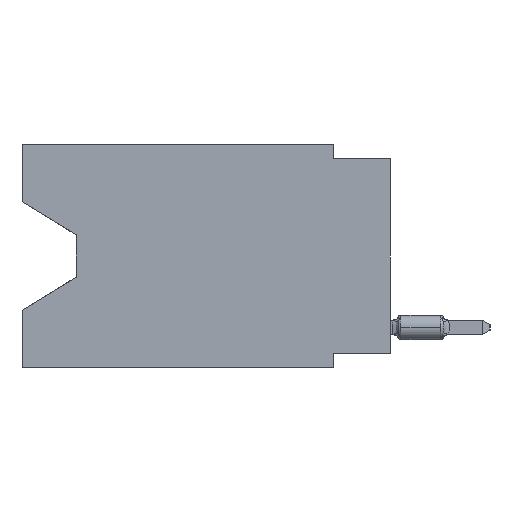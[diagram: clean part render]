
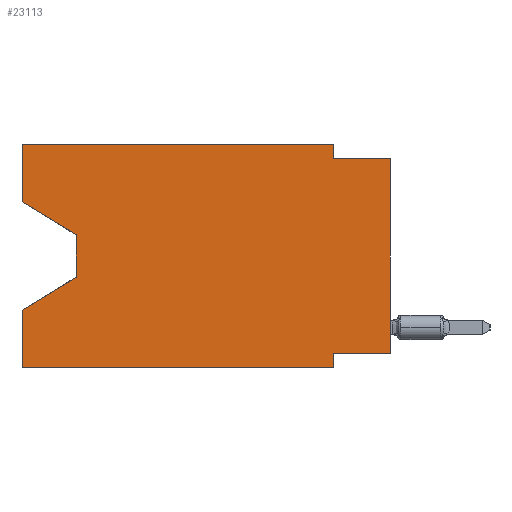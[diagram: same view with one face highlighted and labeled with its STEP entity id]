
A CAD part, left-side view. The second image highlights one B-rep face of the part: STEP entity #23113.
In plain terms, the highlighted planar face has unit normal (-1, 0, 0).
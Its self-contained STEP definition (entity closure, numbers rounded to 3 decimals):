
#590 = VECTOR ( 'NONE', #9091, 1000. ) ;
#1572 = VERTEX_POINT ( 'NONE', #11449 ) ;
#1670 = LINE ( 'NONE', #17598, #19760 ) ;
#2227 = CARTESIAN_POINT ( 'NONE',  ( 0., 0., 0. ) ) ;
#2711 = VECTOR ( 'NONE', #23779, 1000. ) ;
#2842 = DIRECTION ( 'NONE',  ( 0., -1., 0. ) ) ;
#3525 = LINE ( 'NONE', #7686, #2711 ) ;
#3571 = DIRECTION ( 'NONE',  ( 0., 0., -1. ) ) ;
#3828 = ORIENTED_EDGE ( 'NONE', *, *, #14545, .F. ) ;
#3966 = DIRECTION ( 'NONE',  ( 0., 0., 1. ) ) ;
#4262 = EDGE_CURVE ( 'NONE', #13019, #16238, #15889, .T. ) ;
#4271 = CARTESIAN_POINT ( 'NONE',  ( 0., 16.383, -2.546 ) ) ;
#4571 = CARTESIAN_POINT ( 'NONE',  ( 0., 2.54, 0. ) ) ;
#4600 = EDGE_CURVE ( 'NONE', #20387, #22314, #3525, .T. ) ;
#4717 = CARTESIAN_POINT ( 'NONE',  ( 0., 0., -9.271 ) ) ;
#4892 = EDGE_LOOP ( 'NONE', ( #18531, #23934, #24945, #11425, #24817, #5086, #17819, #14226, #20043, #3828, #9235, #13621 ) ) ;
#5086 = ORIENTED_EDGE ( 'NONE', *, *, #4600, .F. ) ;
#5108 = DIRECTION ( 'NONE',  ( 0., 0., -1. ) ) ;
#5160 = CARTESIAN_POINT ( 'NONE',  ( 0., 2.54, -0.635 ) ) ;
#5373 = EDGE_CURVE ( 'NONE', #19283, #24603, #5994, .T. ) ;
#5994 = LINE ( 'NONE', #12174, #19385 ) ;
#5995 = CARTESIAN_POINT ( 'NONE',  ( 0., 16.383, -9.906 ) ) ;
#6090 = LINE ( 'NONE', #13865, #24617 ) ;
#6990 = PLANE ( 'NONE',  #14774 ) ;
#7365 = CARTESIAN_POINT ( 'NONE',  ( 0., 0., -0.635 ) ) ;
#7686 = CARTESIAN_POINT ( 'NONE',  ( 0., 2.54, -9.906 ) ) ;
#8246 = LINE ( 'NONE', #12695, #17704 ) ;
#8514 = VERTEX_POINT ( 'NONE', #7365 ) ;
#8812 = VECTOR ( 'NONE', #2842, 1000. ) ;
#9091 = DIRECTION ( 'NONE',  ( 0., 0., -1. ) ) ;
#9235 = ORIENTED_EDGE ( 'NONE', *, *, #19040, .F. ) ;
#9449 = CARTESIAN_POINT ( 'NONE',  ( 0., 16.383, 0. ) ) ;
#9459 = CARTESIAN_POINT ( 'NONE',  ( 0., 16.383, -9.906 ) ) ;
#9514 = VERTEX_POINT ( 'NONE', #24163 ) ;
#9775 = CARTESIAN_POINT ( 'NONE',  ( 0., 16.383, 0. ) ) ;
#9853 = EDGE_CURVE ( 'NONE', #26405, #9514, #11946, .T. ) ;
#9972 = CARTESIAN_POINT ( 'NONE',  ( 0., 2.54, -9.271 ) ) ;
#10276 = EDGE_CURVE ( 'NONE', #10586, #8514, #21690, .T. ) ;
#10586 = VERTEX_POINT ( 'NONE', #5160 ) ;
#11425 = ORIENTED_EDGE ( 'NONE', *, *, #9853, .F. ) ;
#11449 = CARTESIAN_POINT ( 'NONE',  ( 0., 2.54, 0. ) ) ;
#11501 = LINE ( 'NONE', #9459, #8812 ) ;
#11634 = VECTOR ( 'NONE', #23858, 1000. ) ;
#11694 = CARTESIAN_POINT ( 'NONE',  ( 0., 0., -9.271 ) ) ;
#11946 = LINE ( 'NONE', #9775, #11634 ) ;
#12174 = CARTESIAN_POINT ( 'NONE',  ( 0., 13.97, -4.013 ) ) ;
#12695 = CARTESIAN_POINT ( 'NONE',  ( 0., 16.383, -2.546 ) ) ;
#12700 = VECTOR ( 'NONE', #3966, 1000. ) ;
#13019 = VERTEX_POINT ( 'NONE', #4271 ) ;
#13621 = ORIENTED_EDGE ( 'NONE', *, *, #4262, .F. ) ;
#13865 = CARTESIAN_POINT ( 'NONE',  ( 0., 16.383, 0. ) ) ;
#14111 = EDGE_CURVE ( 'NONE', #13019, #19283, #8246, .T. ) ;
#14156 = LINE ( 'NONE', #2227, #12700 ) ;
#14226 = ORIENTED_EDGE ( 'NONE', *, *, #24074, .T. ) ;
#14545 = EDGE_CURVE ( 'NONE', #1572, #10586, #23308, .T. ) ;
#14774 = AXIS2_PLACEMENT_3D ( 'NONE', #25496, #23464, #5108 ) ;
#15572 = LINE ( 'NONE', #11694, #23337 ) ;
#15725 = VERTEX_POINT ( 'NONE', #4717 ) ;
#15889 = LINE ( 'NONE', #9449, #21069 ) ;
#15907 = DIRECTION ( 'NONE',  ( 0., -1., 0. ) ) ;
#16046 = DIRECTION ( 'NONE',  ( 0., 0., 1. ) ) ;
#16238 = VERTEX_POINT ( 'NONE', #25583 ) ;
#16348 = VECTOR ( 'NONE', #15907, 1000. ) ;
#17598 = CARTESIAN_POINT ( 'NONE',  ( 0., 13.97, -5.893 ) ) ;
#17704 = VECTOR ( 'NONE', #22990, 1000. ) ;
#17819 = ORIENTED_EDGE ( 'NONE', *, *, #19540, .F. ) ;
#17880 = DIRECTION ( 'NONE',  ( 0., -1., 0. ) ) ;
#18502 = CARTESIAN_POINT ( 'NONE',  ( 0., 13.97, -5.893 ) ) ;
#18531 = ORIENTED_EDGE ( 'NONE', *, *, #14111, .T. ) ;
#19040 = EDGE_CURVE ( 'NONE', #16238, #1572, #6090, .T. ) ;
#19080 = CARTESIAN_POINT ( 'NONE',  ( 0., 13.97, -4.013 ) ) ;
#19283 = VERTEX_POINT ( 'NONE', #19080 ) ;
#19385 = VECTOR ( 'NONE', #3571, 1000. ) ;
#19540 = EDGE_CURVE ( 'NONE', #15725, #20387, #15572, .T. ) ;
#19611 = DIRECTION ( 'NONE',  ( 0., 0.855, -0.519 ) ) ;
#19747 = EDGE_CURVE ( 'NONE', #26405, #22314, #11501, .T. ) ;
#19760 = VECTOR ( 'NONE', #19611, 1000. ) ;
#19855 = DIRECTION ( 'NONE',  ( 0., 1., 0. ) ) ;
#20043 = ORIENTED_EDGE ( 'NONE', *, *, #10276, .F. ) ;
#20387 = VERTEX_POINT ( 'NONE', #9972 ) ;
#21069 = VECTOR ( 'NONE', #16046, 1000. ) ;
#21690 = LINE ( 'NONE', #21939, #16348 ) ;
#21939 = CARTESIAN_POINT ( 'NONE',  ( 0., 0., -0.635 ) ) ;
#21979 = CARTESIAN_POINT ( 'NONE',  ( 0., 2.54, -9.906 ) ) ;
#22314 = VERTEX_POINT ( 'NONE', #21979 ) ;
#22990 = DIRECTION ( 'NONE',  ( 0., -0.855, -0.519 ) ) ;
#23113 = ADVANCED_FACE ( 'NONE', ( #25352 ), #6990, .F. ) ;
#23308 = LINE ( 'NONE', #4571, #590 ) ;
#23337 = VECTOR ( 'NONE', #19855, 1000. ) ;
#23464 = DIRECTION ( 'NONE',  ( 1., 0., 0. ) ) ;
#23779 = DIRECTION ( 'NONE',  ( 0., 0., -1. ) ) ;
#23858 = DIRECTION ( 'NONE',  ( 0., 0., 1. ) ) ;
#23934 = ORIENTED_EDGE ( 'NONE', *, *, #5373, .T. ) ;
#24074 = EDGE_CURVE ( 'NONE', #15725, #8514, #14156, .T. ) ;
#24163 = CARTESIAN_POINT ( 'NONE',  ( 0., 16.383, -7.36 ) ) ;
#24603 = VERTEX_POINT ( 'NONE', #18502 ) ;
#24617 = VECTOR ( 'NONE', #17880, 1000. ) ;
#24817 = ORIENTED_EDGE ( 'NONE', *, *, #19747, .T. ) ;
#24945 = ORIENTED_EDGE ( 'NONE', *, *, #25619, .T. ) ;
#25352 = FACE_OUTER_BOUND ( 'NONE', #4892, .T. ) ;
#25496 = CARTESIAN_POINT ( 'NONE',  ( 0., 16.383, 0. ) ) ;
#25583 = CARTESIAN_POINT ( 'NONE',  ( 0., 16.383, 0. ) ) ;
#25619 = EDGE_CURVE ( 'NONE', #24603, #9514, #1670, .T. ) ;
#26405 = VERTEX_POINT ( 'NONE', #5995 ) ;
